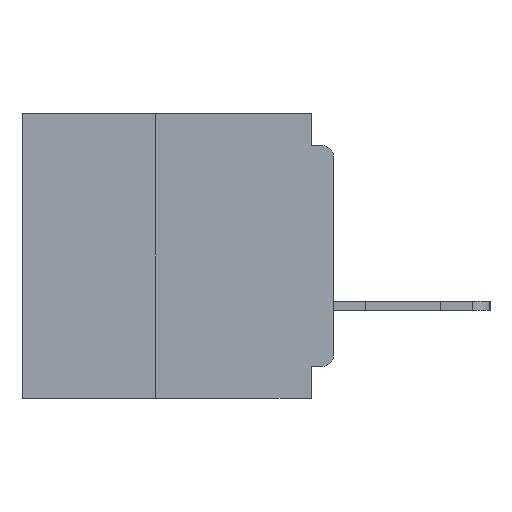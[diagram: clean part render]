
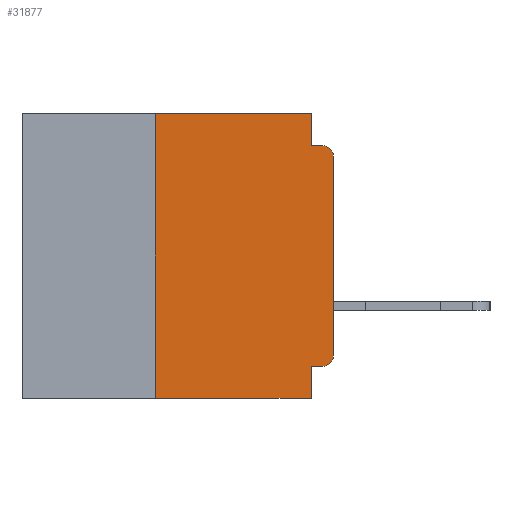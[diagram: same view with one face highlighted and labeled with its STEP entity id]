
A CAD part, left-side view. The second image highlights one B-rep face of the part: STEP entity #31877.
In plain terms, the highlighted planar face has unit normal (-1, 0, 0).
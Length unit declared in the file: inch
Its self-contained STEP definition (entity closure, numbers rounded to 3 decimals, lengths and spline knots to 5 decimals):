
#112 = FACE_OUTER_BOUND ( 'NONE', #21360, .T. ) ;
#243 = CIRCLE ( 'NONE', #52057, 0.015 ) ;
#429 = AXIS2_PLACEMENT_3D ( 'NONE', #45279, #17471, #49924 ) ;
#1348 = LINE ( 'NONE', #32537, #13716 ) ;
#2528 = CARTESIAN_POINT ( 'NONE',  ( 0., 0., -0.06 ) ) ;
#2566 = EDGE_CURVE ( 'NONE', #28301, #5050, #7749, .T. ) ;
#4277 = EDGE_CURVE ( 'NONE', #42313, #16511, #6071, .T. ) ;
#4438 = VECTOR ( 'NONE', #13243, 39.37008 ) ;
#4829 = VECTOR ( 'NONE', #24055, 39.37008 ) ;
#5050 = VERTEX_POINT ( 'NONE', #60042 ) ;
#5776 = CARTESIAN_POINT ( 'NONE',  ( 0., 0.437, 0. ) ) ;
#6071 = CIRCLE ( 'NONE', #429, 0.015 ) ;
#7749 = LINE ( 'NONE', #30709, #4829 ) ;
#7923 = VECTOR ( 'NONE', #29456, 39.37008 ) ;
#8353 = VERTEX_POINT ( 'NONE', #44927 ) ;
#9161 = CARTESIAN_POINT ( 'NONE',  ( 0., 0., 0. ) ) ;
#9434 = DIRECTION ( 'NONE',  ( 0., 1., 0. ) ) ;
#10359 = ORIENTED_EDGE ( 'NONE', *, *, #2566, .F. ) ;
#10444 = DIRECTION ( 'NONE',  ( 1., 0., 0. ) ) ;
#10920 = ORIENTED_EDGE ( 'NONE', *, *, #17960, .T. ) ;
#11018 = CARTESIAN_POINT ( 'NONE',  ( 0., 0.015, -0.06 ) ) ;
#11200 = CARTESIAN_POINT ( 'NONE',  ( 0., 0.031, 0. ) ) ;
#11254 = VERTEX_POINT ( 'NONE', #50424 ) ;
#13243 = DIRECTION ( 'NONE',  ( 0., -1., 0. ) ) ;
#13716 = VECTOR ( 'NONE', #9434, 39.37008 ) ;
#14350 = CARTESIAN_POINT ( 'NONE',  ( 0., 0.015, -0.355 ) ) ;
#15161 = EDGE_CURVE ( 'NONE', #34836, #36409, #24625, .T. ) ;
#15709 = DIRECTION ( 'NONE',  ( 0., 0., -1. ) ) ;
#16511 = VERTEX_POINT ( 'NONE', #56425 ) ;
#17471 = DIRECTION ( 'NONE',  ( -1., 0., 0. ) ) ;
#17756 = ORIENTED_EDGE ( 'NONE', *, *, #32243, .F. ) ;
#17960 = EDGE_CURVE ( 'NONE', #34273, #11254, #243, .T. ) ;
#18940 = CARTESIAN_POINT ( 'NONE',  ( 0., 0.031, -0.4 ) ) ;
#20281 = EDGE_CURVE ( 'NONE', #16511, #34273, #53109, .T. ) ;
#21360 = EDGE_LOOP ( 'NONE', ( #22624, #10920, #17756, #10359, #56887, #56098, #58120, #56130, #52515, #51247 ) ) ;
#22045 = CARTESIAN_POINT ( 'NONE',  ( 0., 0.25, 0. ) ) ;
#22624 = ORIENTED_EDGE ( 'NONE', *, *, #20281, .T. ) ;
#24055 = DIRECTION ( 'NONE',  ( 0., 0., -1. ) ) ;
#24625 = LINE ( 'NONE', #36967, #60029 ) ;
#24822 = VECTOR ( 'NONE', #26011, 39.37008 ) ;
#26011 = DIRECTION ( 'NONE',  ( 0., -1., 0. ) ) ;
#28301 = VERTEX_POINT ( 'NONE', #11200 ) ;
#28535 = VECTOR ( 'NONE', #59873, 39.37008 ) ;
#29456 = DIRECTION ( 'NONE',  ( 0., 0., 1. ) ) ;
#30709 = CARTESIAN_POINT ( 'NONE',  ( 0., 0.031, 0. ) ) ;
#31144 = EDGE_CURVE ( 'NONE', #42218, #28301, #40927, .T. ) ;
#31877 = ADVANCED_FACE ( 'NONE', ( #112 ), #33568, .F. ) ;
#32243 = EDGE_CURVE ( 'NONE', #5050, #11254, #40070, .T. ) ;
#32409 = AXIS2_PLACEMENT_3D ( 'NONE', #5776, #10444, #42956 ) ;
#32537 = CARTESIAN_POINT ( 'NONE',  ( 0., 0., -0.355 ) ) ;
#33568 = PLANE ( 'NONE',  #32409 ) ;
#33599 = EDGE_CURVE ( 'NONE', #42313, #34836, #1348, .T. ) ;
#34273 = VERTEX_POINT ( 'NONE', #2528 ) ;
#34530 = CARTESIAN_POINT ( 'NONE',  ( 0., 0.031, -0.355 ) ) ;
#34836 = VERTEX_POINT ( 'NONE', #34530 ) ;
#36409 = VERTEX_POINT ( 'NONE', #18940 ) ;
#36967 = CARTESIAN_POINT ( 'NONE',  ( 0., 0.031, -0.4 ) ) ;
#37156 = LINE ( 'NONE', #53772, #24822 ) ;
#38192 = EDGE_CURVE ( 'NONE', #8353, #42218, #57225, .T. ) ;
#40070 = LINE ( 'NONE', #41061, #4438 ) ;
#40833 = VECTOR ( 'NONE', #50930, 39.37008 ) ;
#40927 = LINE ( 'NONE', #55288, #28535 ) ;
#41061 = CARTESIAN_POINT ( 'NONE',  ( 0., 0., -0.045 ) ) ;
#42218 = VERTEX_POINT ( 'NONE', #22045 ) ;
#42313 = VERTEX_POINT ( 'NONE', #14350 ) ;
#42956 = DIRECTION ( 'NONE',  ( 0., 0., -1. ) ) ;
#43516 = DIRECTION ( 'NONE',  ( -1., 0., 0. ) ) ;
#43789 = EDGE_CURVE ( 'NONE', #8353, #36409, #37156, .T. ) ;
#44927 = CARTESIAN_POINT ( 'NONE',  ( 0., 0.25, -0.4 ) ) ;
#45279 = CARTESIAN_POINT ( 'NONE',  ( 0., 0.015, -0.34 ) ) ;
#49924 = DIRECTION ( 'NONE',  ( 0., 0., -1. ) ) ;
#50424 = CARTESIAN_POINT ( 'NONE',  ( 0., 0.015, -0.045 ) ) ;
#50930 = DIRECTION ( 'NONE',  ( 0., 0., 1. ) ) ;
#51247 = ORIENTED_EDGE ( 'NONE', *, *, #4277, .T. ) ;
#52057 = AXIS2_PLACEMENT_3D ( 'NONE', #11018, #43516, #15709 ) ;
#52515 = ORIENTED_EDGE ( 'NONE', *, *, #33599, .F. ) ;
#52556 = CARTESIAN_POINT ( 'NONE',  ( 0., 0.25, -0.4 ) ) ;
#53109 = LINE ( 'NONE', #9161, #40833 ) ;
#53772 = CARTESIAN_POINT ( 'NONE',  ( 0., 0.437, -0.4 ) ) ;
#55288 = CARTESIAN_POINT ( 'NONE',  ( 0., 0.437, 0. ) ) ;
#56098 = ORIENTED_EDGE ( 'NONE', *, *, #38192, .F. ) ;
#56130 = ORIENTED_EDGE ( 'NONE', *, *, #15161, .F. ) ;
#56425 = CARTESIAN_POINT ( 'NONE',  ( 0., 0., -0.34 ) ) ;
#56887 = ORIENTED_EDGE ( 'NONE', *, *, #31144, .F. ) ;
#57225 = LINE ( 'NONE', #52556, #7923 ) ;
#58120 = ORIENTED_EDGE ( 'NONE', *, *, #43789, .T. ) ;
#59873 = DIRECTION ( 'NONE',  ( 0., -1., 0. ) ) ;
#59950 = DIRECTION ( 'NONE',  ( 0., 0., -1. ) ) ;
#60029 = VECTOR ( 'NONE', #59950, 39.37008 ) ;
#60042 = CARTESIAN_POINT ( 'NONE',  ( 0., 0.031, -0.045 ) ) ;
